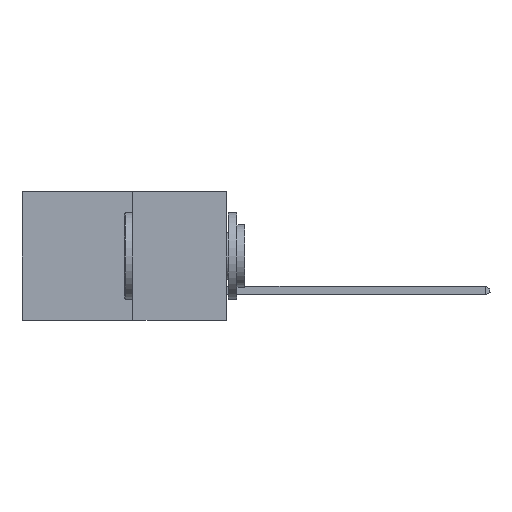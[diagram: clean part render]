
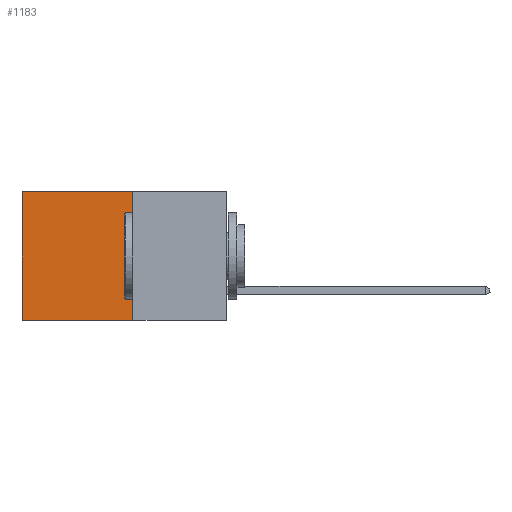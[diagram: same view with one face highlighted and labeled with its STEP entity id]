
A CAD part, left-side view. The second image highlights one B-rep face of the part: STEP entity #1183.
In plain terms, the highlighted planar face has unit normal (-1, 0, 0).
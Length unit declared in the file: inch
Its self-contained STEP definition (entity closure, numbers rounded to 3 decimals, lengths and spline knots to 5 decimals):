
#488 = VERTEX_POINT ( 'NONE', #1037 ) ;
#1037 = CARTESIAN_POINT ( 'NONE',  ( 0.277, 0.59, 0. ) ) ;
#1183 = ADVANCED_FACE ( 'NONE', ( #3098 ), #18621, .F. ) ;
#3098 = FACE_OUTER_BOUND ( 'NONE', #7048, .T. ) ;
#3369 = CARTESIAN_POINT ( 'NONE',  ( 0.277, 0.27, -0.37 ) ) ;
#5669 = VECTOR ( 'NONE', #10115, 39.37008 ) ;
#5729 = DIRECTION ( 'NONE',  ( 0., 1., 0. ) ) ;
#6659 = VERTEX_POINT ( 'NONE', #3369 ) ;
#7048 = EDGE_LOOP ( 'NONE', ( #23109, #17393, #12837, #13138 ) ) ;
#7191 = EDGE_CURVE ( 'NONE', #488, #16311, #12174, .T. ) ;
#8363 = CARTESIAN_POINT ( 'NONE',  ( 0.277, 0.27, -0.37 ) ) ;
#9042 = LINE ( 'NONE', #18174, #23914 ) ;
#10115 = DIRECTION ( 'NONE',  ( 0., 1., 0. ) ) ;
#12174 = LINE ( 'NONE', #25843, #16920 ) ;
#12837 = ORIENTED_EDGE ( 'NONE', *, *, #20790, .F. ) ;
#13138 = ORIENTED_EDGE ( 'NONE', *, *, #14334, .T. ) ;
#13859 = CARTESIAN_POINT ( 'NONE',  ( 0.277, 0.27, 0. ) ) ;
#14334 = EDGE_CURVE ( 'NONE', #14867, #488, #18855, .T. ) ;
#14680 = CARTESIAN_POINT ( 'NONE',  ( 0.277, 0.59, -0.37 ) ) ;
#14867 = VERTEX_POINT ( 'NONE', #15536 ) ;
#15536 = CARTESIAN_POINT ( 'NONE',  ( 0.277, 0.27, 0. ) ) ;
#16311 = VERTEX_POINT ( 'NONE', #14680 ) ;
#16920 = VECTOR ( 'NONE', #26391, 39.37008 ) ;
#17393 = ORIENTED_EDGE ( 'NONE', *, *, #26069, .F. ) ;
#18174 = CARTESIAN_POINT ( 'NONE',  ( 0.277, 0.27, -0.37 ) ) ;
#18621 = PLANE ( 'NONE',  #25521 ) ;
#18855 = LINE ( 'NONE', #13859, #24209 ) ;
#20232 = CARTESIAN_POINT ( 'NONE',  ( 0.277, 0.27, -0.37 ) ) ;
#20299 = DIRECTION ( 'NONE',  ( 0., 0., -1. ) ) ;
#20317 = DIRECTION ( 'NONE',  ( 1., 0., 0. ) ) ;
#20790 = EDGE_CURVE ( 'NONE', #14867, #6659, #9042, .T. ) ;
#21908 = LINE ( 'NONE', #20232, #5669 ) ;
#23109 = ORIENTED_EDGE ( 'NONE', *, *, #7191, .T. ) ;
#23914 = VECTOR ( 'NONE', #26287, 39.37008 ) ;
#24209 = VECTOR ( 'NONE', #5729, 39.37008 ) ;
#25521 = AXIS2_PLACEMENT_3D ( 'NONE', #8363, #20317, #20299 ) ;
#25843 = CARTESIAN_POINT ( 'NONE',  ( 0.277, 0.59, -0.37 ) ) ;
#26069 = EDGE_CURVE ( 'NONE', #6659, #16311, #21908, .T. ) ;
#26287 = DIRECTION ( 'NONE',  ( 0., 0., -1. ) ) ;
#26391 = DIRECTION ( 'NONE',  ( 0., 0., -1. ) ) ;
